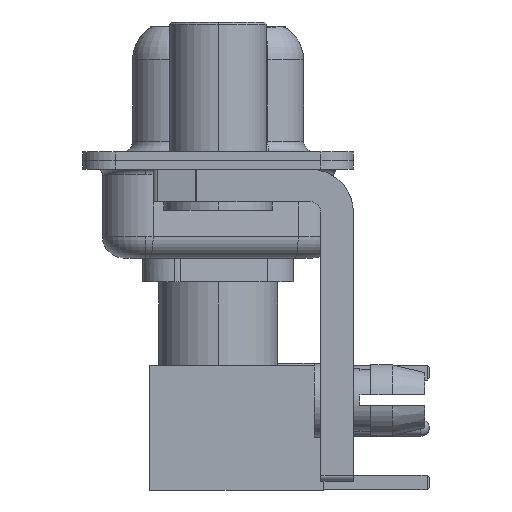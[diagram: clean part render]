
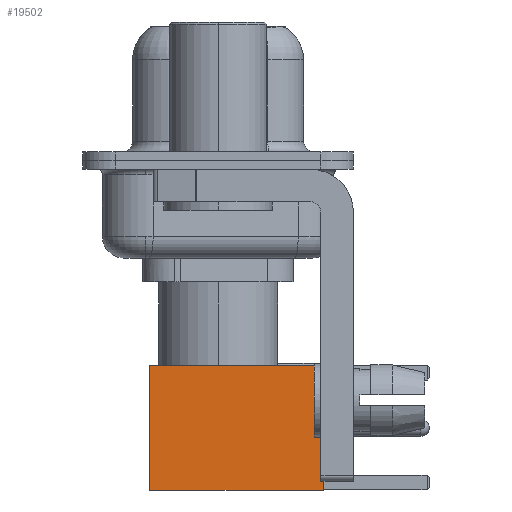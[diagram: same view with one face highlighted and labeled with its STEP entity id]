
A CAD part, left-side view. The second image highlights one B-rep face of the part: STEP entity #19502.
In plain terms, the highlighted face is planar.
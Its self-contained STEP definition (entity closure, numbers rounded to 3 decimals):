
#428 = VECTOR ( 'NONE', #8126, 1000. ) ;
#1257 = VERTEX_POINT ( 'NONE', #17956 ) ;
#1338 = ORIENTED_EDGE ( 'NONE', *, *, #15798, .T. ) ;
#2440 = AXIS2_PLACEMENT_3D ( 'NONE', #19124, #23540, #27788 ) ;
#2857 = EDGE_CURVE ( 'NONE', #1257, #19546, #6191, .T. ) ;
#3244 = VECTOR ( 'NONE', #4145, 1000. ) ;
#3492 = ORIENTED_EDGE ( 'NONE', *, *, #12876, .F. ) ;
#3673 = CARTESIAN_POINT ( 'NONE',  ( 0., 2.875, 0. ) ) ;
#4000 = VECTOR ( 'NONE', #8446, 1000. ) ;
#4145 = DIRECTION ( 'NONE',  ( 0., 0., -1. ) ) ;
#4434 = LINE ( 'NONE', #21706, #428 ) ;
#5229 = CARTESIAN_POINT ( 'NONE',  ( -2.875, 2.875, 0. ) ) ;
#6191 = LINE ( 'NONE', #14808, #4000 ) ;
#6502 = CARTESIAN_POINT ( 'NONE',  ( 2.875, 2.875, 0. ) ) ;
#7357 = ORIENTED_EDGE ( 'NONE', *, *, #2857, .F. ) ;
#8126 = DIRECTION ( 'NONE',  ( -1., 0., 0. ) ) ;
#8422 = CARTESIAN_POINT ( 'NONE',  ( 2.875, 2.875, 0. ) ) ;
#8446 = DIRECTION ( 'NONE',  ( 0., 0., -1. ) ) ;
#9488 = ORIENTED_EDGE ( 'NONE', *, *, #11189, .T. ) ;
#11189 = EDGE_CURVE ( 'NONE', #16286, #19546, #23102, .T. ) ;
#12627 = EDGE_LOOP ( 'NONE', ( #1338, #9488, #7357, #3492 ) ) ;
#12876 = EDGE_CURVE ( 'NONE', #21787, #1257, #4434, .T. ) ;
#14808 = CARTESIAN_POINT ( 'NONE',  ( -2.875, 2.875, 0. ) ) ;
#15798 = EDGE_CURVE ( 'NONE', #21787, #16286, #16891, .T. ) ;
#16286 = VERTEX_POINT ( 'NONE', #6502 ) ;
#16891 = LINE ( 'NONE', #8422, #3244 ) ;
#17956 = CARTESIAN_POINT ( 'NONE',  ( -2.875, 2.875, 8. ) ) ;
#18843 = DIRECTION ( 'NONE',  ( -1., 0., 0. ) ) ;
#19124 = CARTESIAN_POINT ( 'NONE',  ( 2.875, 2.875, 0. ) ) ;
#19226 = VECTOR ( 'NONE', #18843, 1000. ) ;
#19502 = ADVANCED_FACE ( 'NONE', ( #21830 ), #19720, .T. ) ;
#19546 = VERTEX_POINT ( 'NONE', #5229 ) ;
#19720 = PLANE ( 'NONE',  #2440 ) ;
#21706 = CARTESIAN_POINT ( 'NONE',  ( 0., 2.875, 8. ) ) ;
#21787 = VERTEX_POINT ( 'NONE', #25829 ) ;
#21830 = FACE_OUTER_BOUND ( 'NONE', #12627, .T. ) ;
#23102 = LINE ( 'NONE', #3673, #19226 ) ;
#23540 = DIRECTION ( 'NONE',  ( 0., 1., 0. ) ) ;
#25829 = CARTESIAN_POINT ( 'NONE',  ( 2.875, 2.875, 8. ) ) ;
#27788 = DIRECTION ( 'NONE',  ( 0., 0., 1. ) ) ;
